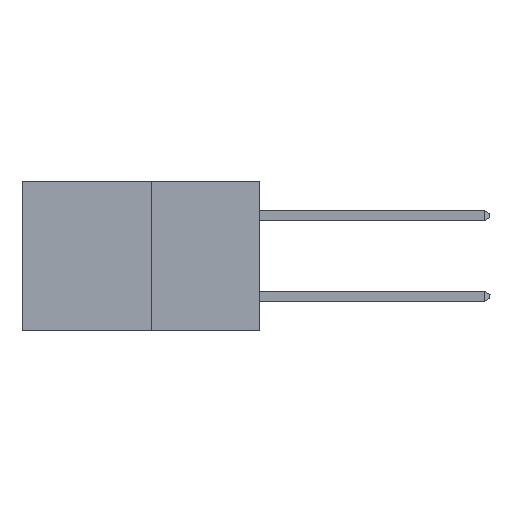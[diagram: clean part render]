
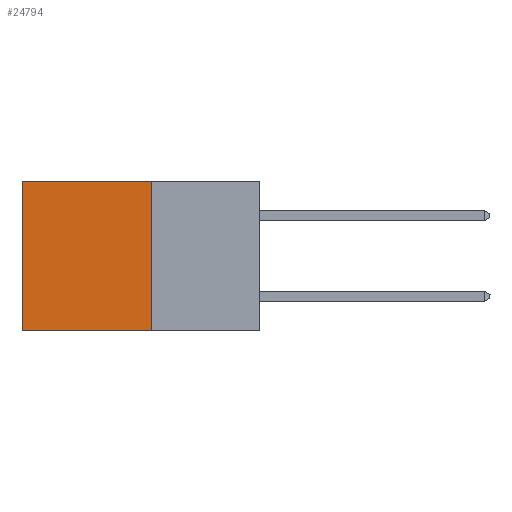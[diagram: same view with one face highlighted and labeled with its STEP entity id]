
A CAD part, left-side view. The second image highlights one B-rep face of the part: STEP entity #24794.
In plain terms, the highlighted planar face has unit normal (-1, 0, 0).
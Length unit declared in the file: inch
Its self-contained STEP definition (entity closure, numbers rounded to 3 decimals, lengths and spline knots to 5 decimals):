
#505 = VECTOR ( 'NONE', #3722, 39.37008 ) ;
#1406 = LINE ( 'NONE', #4165, #6530 ) ;
#2106 = VERTEX_POINT ( 'NONE', #17538 ) ;
#3722 = DIRECTION ( 'NONE',  ( 0., 0., -1. ) ) ;
#3815 = CARTESIAN_POINT ( 'NONE',  ( 0.277, 0.59, -0.37 ) ) ;
#4165 = CARTESIAN_POINT ( 'NONE',  ( 0.277, 0.27, -0.37 ) ) ;
#5044 = CARTESIAN_POINT ( 'NONE',  ( 0.277, 0.59, -0.37 ) ) ;
#6026 = EDGE_CURVE ( 'NONE', #2106, #10087, #24577, .T. ) ;
#6530 = VECTOR ( 'NONE', #23283, 39.37008 ) ;
#7095 = ORIENTED_EDGE ( 'NONE', *, *, #11465, .T. ) ;
#8424 = VECTOR ( 'NONE', #22489, 39.37008 ) ;
#8458 = PLANE ( 'NONE',  #10840 ) ;
#8631 = FACE_OUTER_BOUND ( 'NONE', #19323, .T. ) ;
#8698 = ORIENTED_EDGE ( 'NONE', *, *, #22814, .F. ) ;
#9784 = CARTESIAN_POINT ( 'NONE',  ( 0.277, 0.27, 0. ) ) ;
#10087 = VERTEX_POINT ( 'NONE', #5044 ) ;
#10172 = LINE ( 'NONE', #9784, #20737 ) ;
#10496 = EDGE_CURVE ( 'NONE', #26765, #20290, #1406, .T. ) ;
#10840 = AXIS2_PLACEMENT_3D ( 'NONE', #23248, #25382, #12702 ) ;
#11465 = EDGE_CURVE ( 'NONE', #26765, #2106, #10172, .T. ) ;
#11854 = CARTESIAN_POINT ( 'NONE',  ( 0.277, 0.27, -0.37 ) ) ;
#11869 = DIRECTION ( 'NONE',  ( 0., 1., 0. ) ) ;
#12702 = DIRECTION ( 'NONE',  ( 0., 0., -1. ) ) ;
#15371 = LINE ( 'NONE', #11854, #8424 ) ;
#17001 = CARTESIAN_POINT ( 'NONE',  ( 0.277, 0.27, -0.37 ) ) ;
#17335 = ORIENTED_EDGE ( 'NONE', *, *, #6026, .T. ) ;
#17538 = CARTESIAN_POINT ( 'NONE',  ( 0.277, 0.59, 0. ) ) ;
#17974 = ORIENTED_EDGE ( 'NONE', *, *, #10496, .F. ) ;
#19323 = EDGE_LOOP ( 'NONE', ( #17335, #8698, #17974, #7095 ) ) ;
#20290 = VERTEX_POINT ( 'NONE', #17001 ) ;
#20737 = VECTOR ( 'NONE', #11869, 39.37008 ) ;
#22489 = DIRECTION ( 'NONE',  ( 0., 1., 0. ) ) ;
#22814 = EDGE_CURVE ( 'NONE', #20290, #10087, #15371, .T. ) ;
#23248 = CARTESIAN_POINT ( 'NONE',  ( 0.277, 0.27, -0.37 ) ) ;
#23283 = DIRECTION ( 'NONE',  ( 0., 0., -1. ) ) ;
#24577 = LINE ( 'NONE', #3815, #505 ) ;
#24794 = ADVANCED_FACE ( 'NONE', ( #8631 ), #8458, .F. ) ;
#25382 = DIRECTION ( 'NONE',  ( 1., 0., 0. ) ) ;
#25472 = CARTESIAN_POINT ( 'NONE',  ( 0.277, 0.27, 0. ) ) ;
#26765 = VERTEX_POINT ( 'NONE', #25472 ) ;
